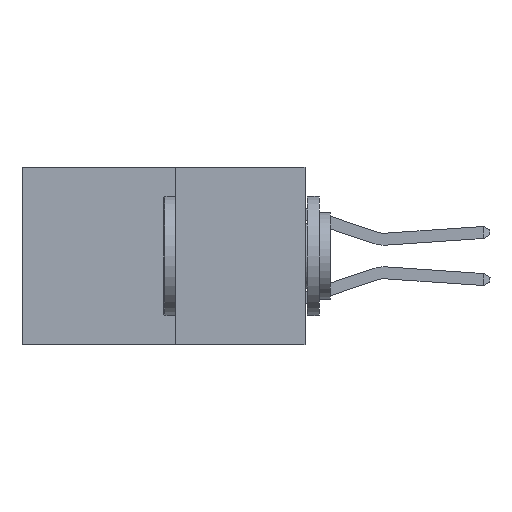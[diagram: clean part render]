
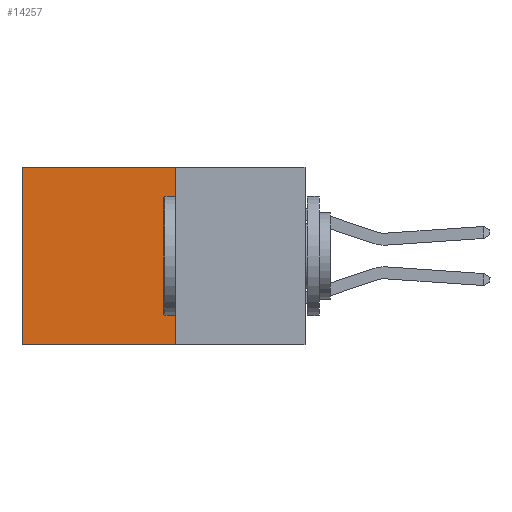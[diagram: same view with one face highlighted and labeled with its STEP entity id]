
A CAD part, left-side view. The second image highlights one B-rep face of the part: STEP entity #14257.
In plain terms, the highlighted planar face has unit normal (-1, 0, 0).
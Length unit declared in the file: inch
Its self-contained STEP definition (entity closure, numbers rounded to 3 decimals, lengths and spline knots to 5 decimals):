
#70 = AXIS2_PLACEMENT_3D ( 'NONE', #11556, #13298, #2876 ) ;
#1505 = LINE ( 'NONE', #7986, #20586 ) ;
#2299 = LINE ( 'NONE', #18717, #6419 ) ;
#2834 = EDGE_CURVE ( 'NONE', #20165, #11964, #1505, .T. ) ;
#2876 = DIRECTION ( 'NONE',  ( 0., 0., -1. ) ) ;
#4088 = FACE_OUTER_BOUND ( 'NONE', #22323, .T. ) ;
#5073 = CARTESIAN_POINT ( 'NONE',  ( 0.277, 0.27, -0.37 ) ) ;
#6031 = LINE ( 'NONE', #21897, #14726 ) ;
#6419 = VECTOR ( 'NONE', #13522, 39.37008 ) ;
#6692 = EDGE_CURVE ( 'NONE', #16017, #11964, #6031, .T. ) ;
#7986 = CARTESIAN_POINT ( 'NONE',  ( 0.277, 0.27, -0.37 ) ) ;
#8033 = ORIENTED_EDGE ( 'NONE', *, *, #2834, .F. ) ;
#9239 = EDGE_CURVE ( 'NONE', #14233, #20165, #14913, .T. ) ;
#10269 = DIRECTION ( 'NONE',  ( 0., 0., -1. ) ) ;
#11556 = CARTESIAN_POINT ( 'NONE',  ( 0.277, 0.27, -0.37 ) ) ;
#11911 = CARTESIAN_POINT ( 'NONE',  ( 0.277, 0.59, 0. ) ) ;
#11964 = VERTEX_POINT ( 'NONE', #19660 ) ;
#12152 = DIRECTION ( 'NONE',  ( 0., 1., 0. ) ) ;
#13298 = DIRECTION ( 'NONE',  ( 1., 0., 0. ) ) ;
#13522 = DIRECTION ( 'NONE',  ( 0., 1., 0. ) ) ;
#14233 = VERTEX_POINT ( 'NONE', #14994 ) ;
#14257 = ADVANCED_FACE ( 'NONE', ( #4088 ), #21977, .F. ) ;
#14726 = VECTOR ( 'NONE', #21859, 39.37008 ) ;
#14913 = LINE ( 'NONE', #18401, #17931 ) ;
#14994 = CARTESIAN_POINT ( 'NONE',  ( 0.277, 0.27, 0. ) ) ;
#16017 = VERTEX_POINT ( 'NONE', #11911 ) ;
#17931 = VECTOR ( 'NONE', #10269, 39.37008 ) ;
#18105 = ORIENTED_EDGE ( 'NONE', *, *, #20048, .T. ) ;
#18401 = CARTESIAN_POINT ( 'NONE',  ( 0.277, 0.27, -0.37 ) ) ;
#18717 = CARTESIAN_POINT ( 'NONE',  ( 0.277, 0.27, 0. ) ) ;
#19660 = CARTESIAN_POINT ( 'NONE',  ( 0.277, 0.59, -0.37 ) ) ;
#20048 = EDGE_CURVE ( 'NONE', #14233, #16017, #2299, .T. ) ;
#20165 = VERTEX_POINT ( 'NONE', #5073 ) ;
#20586 = VECTOR ( 'NONE', #12152, 39.37008 ) ;
#21276 = ORIENTED_EDGE ( 'NONE', *, *, #9239, .F. ) ;
#21505 = ORIENTED_EDGE ( 'NONE', *, *, #6692, .T. ) ;
#21859 = DIRECTION ( 'NONE',  ( 0., 0., -1. ) ) ;
#21897 = CARTESIAN_POINT ( 'NONE',  ( 0.277, 0.59, -0.37 ) ) ;
#21977 = PLANE ( 'NONE',  #70 ) ;
#22323 = EDGE_LOOP ( 'NONE', ( #21505, #8033, #21276, #18105 ) ) ;
